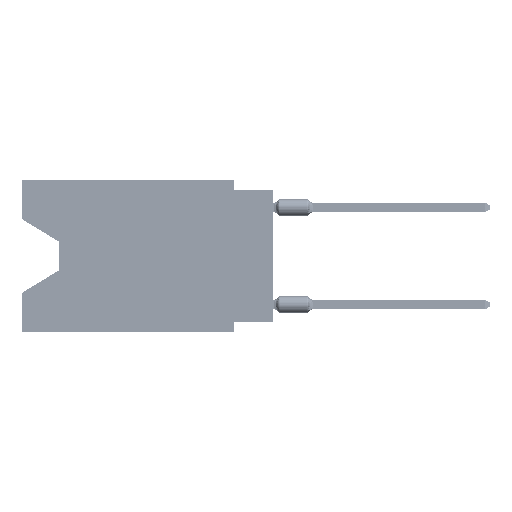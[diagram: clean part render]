
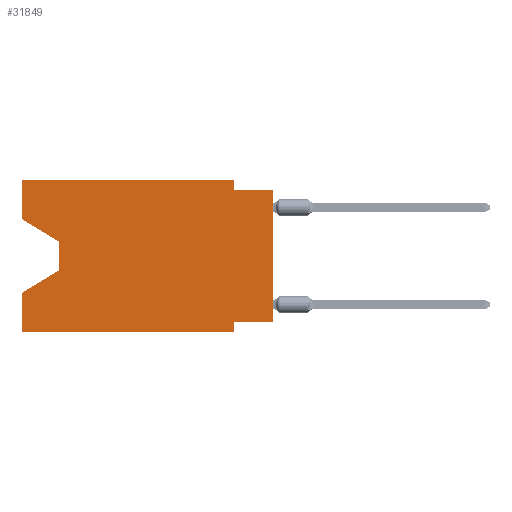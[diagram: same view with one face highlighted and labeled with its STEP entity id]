
A CAD part, left-side view. The second image highlights one B-rep face of the part: STEP entity #31849.
In plain terms, the highlighted planar face has unit normal (-1, 0, 0).
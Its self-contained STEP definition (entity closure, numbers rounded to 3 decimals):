
#11 = DIRECTION ( 'NONE',  ( 0., 0.855, -0.519 ) ) ;
#881 = EDGE_CURVE ( 'NONE', #10145, #3558, #27223, .T. ) ;
#1988 = EDGE_CURVE ( 'NONE', #56649, #27804, #50999, .T. ) ;
#2720 = VERTEX_POINT ( 'NONE', #36633 ) ;
#3558 = VERTEX_POINT ( 'NONE', #54595 ) ;
#3891 = FACE_OUTER_BOUND ( 'NONE', #27245, .T. ) ;
#4544 = CARTESIAN_POINT ( 'NONE',  ( 0., 16.383, 0. ) ) ;
#4788 = EDGE_CURVE ( 'NONE', #2720, #72166, #55415, .T. ) ;
#4799 = LINE ( 'NONE', #55089, #61658 ) ;
#6850 = VECTOR ( 'NONE', #20165, 1000. ) ;
#9994 = DIRECTION ( 'NONE',  ( 0., 0., -1. ) ) ;
#10061 = DIRECTION ( 'NONE',  ( 0., 1., 0. ) ) ;
#10145 = VERTEX_POINT ( 'NONE', #23696 ) ;
#10186 = CARTESIAN_POINT ( 'NONE',  ( 0., 13.97, -4.013 ) ) ;
#10387 = EDGE_CURVE ( 'NONE', #56649, #33321, #16713, .T. ) ;
#11555 = EDGE_CURVE ( 'NONE', #3558, #77826, #78445, .T. ) ;
#12368 = CARTESIAN_POINT ( 'NONE',  ( 0., 16.383, -7.36 ) ) ;
#12390 = ORIENTED_EDGE ( 'NONE', *, *, #4788, .F. ) ;
#13668 = EDGE_CURVE ( 'NONE', #21676, #32758, #40885, .T. ) ;
#16076 = VECTOR ( 'NONE', #59471, 1000. ) ;
#16713 = LINE ( 'NONE', #40654, #24656 ) ;
#17252 = LINE ( 'NONE', #54555, #16076 ) ;
#17888 = LINE ( 'NONE', #55594, #76643 ) ;
#18044 = ORIENTED_EDGE ( 'NONE', *, *, #42091, .T. ) ;
#18213 = ORIENTED_EDGE ( 'NONE', *, *, #73479, .T. ) ;
#19507 = VERTEX_POINT ( 'NONE', #25092 ) ;
#20165 = DIRECTION ( 'NONE',  ( 0., -1., 0. ) ) ;
#21172 = DIRECTION ( 'NONE',  ( 0., -0.855, -0.519 ) ) ;
#21676 = VERTEX_POINT ( 'NONE', #49415 ) ;
#23659 = CARTESIAN_POINT ( 'NONE',  ( 0., 16.383, 0. ) ) ;
#23696 = CARTESIAN_POINT ( 'NONE',  ( 0., 16.383, -2.546 ) ) ;
#24448 = DIRECTION ( 'NONE',  ( 1., 0., 0. ) ) ;
#24656 = VECTOR ( 'NONE', #65428, 1000. ) ;
#25092 = CARTESIAN_POINT ( 'NONE',  ( 0., 13.97, -5.893 ) ) ;
#27223 = LINE ( 'NONE', #39774, #65020 ) ;
#27245 = EDGE_LOOP ( 'NONE', ( #18213, #18044, #36398, #49299, #55529, #77028, #42264, #33921, #12390, #57612, #60620, #47293 ) ) ;
#27388 = VECTOR ( 'NONE', #72740, 1000. ) ;
#27804 = VERTEX_POINT ( 'NONE', #37600 ) ;
#28672 = PLANE ( 'NONE',  #77685 ) ;
#29554 = CARTESIAN_POINT ( 'NONE',  ( 0., 2.54, -9.271 ) ) ;
#31849 = ADVANCED_FACE ( 'NONE', ( #3891 ), #28672, .F. ) ;
#32486 = DIRECTION ( 'NONE',  ( 0., 0., 1. ) ) ;
#32758 = VERTEX_POINT ( 'NONE', #29554 ) ;
#33321 = VERTEX_POINT ( 'NONE', #12368 ) ;
#33632 = CARTESIAN_POINT ( 'NONE',  ( 0., 16.383, -9.906 ) ) ;
#33921 = ORIENTED_EDGE ( 'NONE', *, *, #47530, .T. ) ;
#34491 = CARTESIAN_POINT ( 'NONE',  ( 0., 0., -0.635 ) ) ;
#36398 = ORIENTED_EDGE ( 'NONE', *, *, #78727, .T. ) ;
#36633 = CARTESIAN_POINT ( 'NONE',  ( 0., 2.54, -0.635 ) ) ;
#37600 = CARTESIAN_POINT ( 'NONE',  ( 0., 2.54, -9.906 ) ) ;
#37912 = VECTOR ( 'NONE', #76832, 1000. ) ;
#38259 = LINE ( 'NONE', #57724, #37912 ) ;
#38422 = CARTESIAN_POINT ( 'NONE',  ( 0., 0., -0.635 ) ) ;
#39774 = CARTESIAN_POINT ( 'NONE',  ( 0., 16.383, 0. ) ) ;
#39938 = VECTOR ( 'NONE', #21172, 1000. ) ;
#40216 = LINE ( 'NONE', #40623, #39938 ) ;
#40623 = CARTESIAN_POINT ( 'NONE',  ( 0., 16.383, -2.546 ) ) ;
#40654 = CARTESIAN_POINT ( 'NONE',  ( 0., 16.383, 0. ) ) ;
#40885 = LINE ( 'NONE', #65665, #42902 ) ;
#42091 = EDGE_CURVE ( 'NONE', #46054, #19507, #59306, .T. ) ;
#42118 = DIRECTION ( 'NONE',  ( 0., 0., -1. ) ) ;
#42264 = ORIENTED_EDGE ( 'NONE', *, *, #13668, .F. ) ;
#42667 = VECTOR ( 'NONE', #59704, 1000. ) ;
#42902 = VECTOR ( 'NONE', #10061, 1000. ) ;
#46054 = VERTEX_POINT ( 'NONE', #65517 ) ;
#47293 = ORIENTED_EDGE ( 'NONE', *, *, #881, .F. ) ;
#47530 = EDGE_CURVE ( 'NONE', #21676, #72166, #38259, .T. ) ;
#49299 = ORIENTED_EDGE ( 'NONE', *, *, #10387, .F. ) ;
#49415 = CARTESIAN_POINT ( 'NONE',  ( 0., 0., -9.271 ) ) ;
#50999 = LINE ( 'NONE', #56280, #6850 ) ;
#52554 = VECTOR ( 'NONE', #80208, 1000. ) ;
#54555 = CARTESIAN_POINT ( 'NONE',  ( 0., 2.54, -9.906 ) ) ;
#54595 = CARTESIAN_POINT ( 'NONE',  ( 0., 16.383, 0. ) ) ;
#55089 = CARTESIAN_POINT ( 'NONE',  ( 0., 2.54, 0. ) ) ;
#55415 = LINE ( 'NONE', #34491, #52554 ) ;
#55529 = ORIENTED_EDGE ( 'NONE', *, *, #1988, .T. ) ;
#55594 = CARTESIAN_POINT ( 'NONE',  ( 0., 13.97, -5.893 ) ) ;
#56280 = CARTESIAN_POINT ( 'NONE',  ( 0., 16.383, -9.906 ) ) ;
#56649 = VERTEX_POINT ( 'NONE', #33632 ) ;
#57612 = ORIENTED_EDGE ( 'NONE', *, *, #72014, .F. ) ;
#57724 = CARTESIAN_POINT ( 'NONE',  ( 0., 0., 0. ) ) ;
#59306 = LINE ( 'NONE', #10186, #42667 ) ;
#59471 = DIRECTION ( 'NONE',  ( 0., 0., -1. ) ) ;
#59704 = DIRECTION ( 'NONE',  ( 0., 0., -1. ) ) ;
#60620 = ORIENTED_EDGE ( 'NONE', *, *, #11555, .F. ) ;
#61658 = VECTOR ( 'NONE', #42118, 1000. ) ;
#65020 = VECTOR ( 'NONE', #32486, 1000. ) ;
#65428 = DIRECTION ( 'NONE',  ( 0., 0., 1. ) ) ;
#65517 = CARTESIAN_POINT ( 'NONE',  ( 0., 13.97, -4.013 ) ) ;
#65665 = CARTESIAN_POINT ( 'NONE',  ( 0., 0., -9.271 ) ) ;
#66901 = CARTESIAN_POINT ( 'NONE',  ( 0., 2.54, 0. ) ) ;
#68368 = EDGE_CURVE ( 'NONE', #32758, #27804, #17252, .T. ) ;
#72014 = EDGE_CURVE ( 'NONE', #77826, #2720, #4799, .T. ) ;
#72166 = VERTEX_POINT ( 'NONE', #38422 ) ;
#72740 = DIRECTION ( 'NONE',  ( 0., -1., 0. ) ) ;
#73479 = EDGE_CURVE ( 'NONE', #10145, #46054, #40216, .T. ) ;
#76643 = VECTOR ( 'NONE', #11, 1000. ) ;
#76832 = DIRECTION ( 'NONE',  ( 0., 0., 1. ) ) ;
#77028 = ORIENTED_EDGE ( 'NONE', *, *, #68368, .F. ) ;
#77685 = AXIS2_PLACEMENT_3D ( 'NONE', #23659, #24448, #9994 ) ;
#77826 = VERTEX_POINT ( 'NONE', #66901 ) ;
#78445 = LINE ( 'NONE', #4544, #27388 ) ;
#78727 = EDGE_CURVE ( 'NONE', #19507, #33321, #17888, .T. ) ;
#80208 = DIRECTION ( 'NONE',  ( 0., -1., 0. ) ) ;
